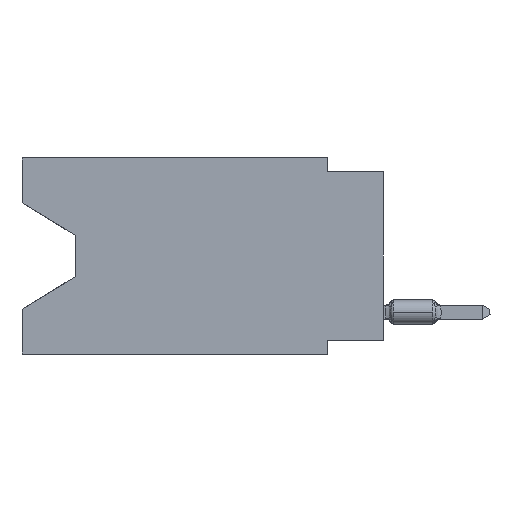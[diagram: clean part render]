
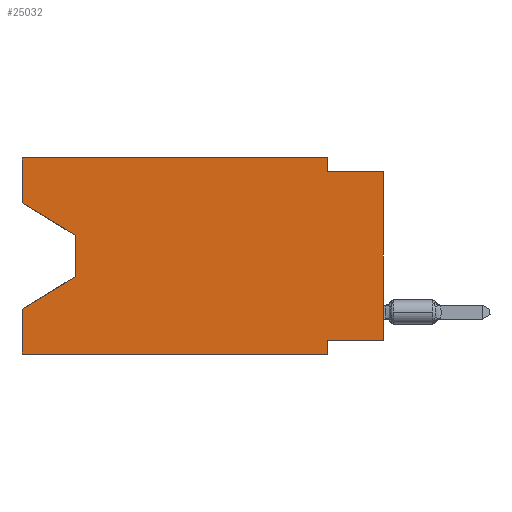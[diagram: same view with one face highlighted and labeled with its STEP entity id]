
A CAD part, left-side view. The second image highlights one B-rep face of the part: STEP entity #25032.
In plain terms, the highlighted planar face has unit normal (-1, 0, 0).
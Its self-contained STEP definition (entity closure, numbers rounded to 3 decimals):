
#564 = ORIENTED_EDGE ( 'NONE', *, *, #35363, .F. ) ;
#917 = CARTESIAN_POINT ( 'NONE',  ( 0., 0., -0.635 ) ) ;
#2523 = VERTEX_POINT ( 'NONE', #16397 ) ;
#2773 = VERTEX_POINT ( 'NONE', #14297 ) ;
#3622 = DIRECTION ( 'NONE',  ( 0., 0., -1. ) ) ;
#4265 = DIRECTION ( 'NONE',  ( 0., 0., -1. ) ) ;
#4941 = EDGE_CURVE ( 'NONE', #18006, #2773, #11663, .T. ) ;
#5604 = EDGE_CURVE ( 'NONE', #17813, #47537, #65028, .T. ) ;
#5994 = AXIS2_PLACEMENT_3D ( 'NONE', #54937, #60303, #4265 ) ;
#6298 = DIRECTION ( 'NONE',  ( 0., 0., -1. ) ) ;
#6953 = DIRECTION ( 'NONE',  ( 0., 0., 1. ) ) ;
#7023 = EDGE_CURVE ( 'NONE', #32067, #2523, #47996, .T. ) ;
#8337 = EDGE_CURVE ( 'NONE', #59845, #60852, #10118, .T. ) ;
#9528 = VECTOR ( 'NONE', #43289, 1000. ) ;
#9959 = VECTOR ( 'NONE', #50485, 1000. ) ;
#10118 = LINE ( 'NONE', #11137, #41432 ) ;
#10743 = EDGE_CURVE ( 'NONE', #2523, #35669, #17047, .T. ) ;
#11085 = DIRECTION ( 'NONE',  ( 0., -1., 0. ) ) ;
#11137 = CARTESIAN_POINT ( 'NONE',  ( 0., 16.383, 0. ) ) ;
#11663 = LINE ( 'NONE', #31842, #63995 ) ;
#11842 = ORIENTED_EDGE ( 'NONE', *, *, #14640, .T. ) ;
#12755 = CARTESIAN_POINT ( 'NONE',  ( 0., 13.97, -3.505 ) ) ;
#14036 = CARTESIAN_POINT ( 'NONE',  ( 0., 2.54, -8.89 ) ) ;
#14253 = CARTESIAN_POINT ( 'NONE',  ( 0., 16.383, -2.038 ) ) ;
#14297 = CARTESIAN_POINT ( 'NONE',  ( 0., 16.383, -6.852 ) ) ;
#14640 = EDGE_CURVE ( 'NONE', #47634, #35669, #22160, .T. ) ;
#15418 = EDGE_CURVE ( 'NONE', #40428, #2773, #18667, .T. ) ;
#16397 = CARTESIAN_POINT ( 'NONE',  ( 0., 2.54, -0.635 ) ) ;
#16847 = CARTESIAN_POINT ( 'NONE',  ( 0., 13.97, -5.385 ) ) ;
#17047 = LINE ( 'NONE', #917, #25531 ) ;
#17813 = VERTEX_POINT ( 'NONE', #23313 ) ;
#18006 = VERTEX_POINT ( 'NONE', #44403 ) ;
#18667 = LINE ( 'NONE', #55518, #9959 ) ;
#20859 = LINE ( 'NONE', #32596, #36740 ) ;
#22106 = LINE ( 'NONE', #32823, #47673 ) ;
#22160 = LINE ( 'NONE', #37249, #54648 ) ;
#22765 = DIRECTION ( 'NONE',  ( 0., -1., 0. ) ) ;
#23313 = CARTESIAN_POINT ( 'NONE',  ( 0., 2.54, -8.255 ) ) ;
#25032 = ADVANCED_FACE ( 'NONE', ( #45218 ), #55597, .F. ) ;
#25205 = ORIENTED_EDGE ( 'NONE', *, *, #28951, .F. ) ;
#25531 = VECTOR ( 'NONE', #22765, 1000. ) ;
#28951 = EDGE_CURVE ( 'NONE', #47634, #17813, #66301, .T. ) ;
#30199 = CARTESIAN_POINT ( 'NONE',  ( 0., 0., -0.635 ) ) ;
#30381 = LINE ( 'NONE', #14253, #64948 ) ;
#30484 = ORIENTED_EDGE ( 'NONE', *, *, #15418, .T. ) ;
#31383 = CARTESIAN_POINT ( 'NONE',  ( 0., 0., -8.255 ) ) ;
#31407 = ORIENTED_EDGE ( 'NONE', *, *, #8337, .F. ) ;
#31522 = ORIENTED_EDGE ( 'NONE', *, *, #55062, .T. ) ;
#31842 = CARTESIAN_POINT ( 'NONE',  ( 0., 16.383, 0. ) ) ;
#32067 = VERTEX_POINT ( 'NONE', #64496 ) ;
#32596 = CARTESIAN_POINT ( 'NONE',  ( 0., 16.383, 0. ) ) ;
#32823 = CARTESIAN_POINT ( 'NONE',  ( 0., 13.97, -3.505 ) ) ;
#33250 = VECTOR ( 'NONE', #60283, 1000. ) ;
#34015 = ORIENTED_EDGE ( 'NONE', *, *, #7023, .F. ) ;
#35363 = EDGE_CURVE ( 'NONE', #60852, #32067, #20859, .T. ) ;
#35669 = VERTEX_POINT ( 'NONE', #30199 ) ;
#36375 = ORIENTED_EDGE ( 'NONE', *, *, #10743, .F. ) ;
#36387 = ORIENTED_EDGE ( 'NONE', *, *, #5604, .F. ) ;
#36740 = VECTOR ( 'NONE', #11085, 1000. ) ;
#37249 = CARTESIAN_POINT ( 'NONE',  ( 0., 0., 0. ) ) ;
#37597 = LINE ( 'NONE', #58042, #9528 ) ;
#37730 = CARTESIAN_POINT ( 'NONE',  ( 0., 16.383, 0. ) ) ;
#38500 = VECTOR ( 'NONE', #3622, 1000. ) ;
#40428 = VERTEX_POINT ( 'NONE', #16847 ) ;
#40830 = CARTESIAN_POINT ( 'NONE',  ( 0., 0., -8.255 ) ) ;
#41432 = VECTOR ( 'NONE', #47410, 1000. ) ;
#42965 = CARTESIAN_POINT ( 'NONE',  ( 0., 2.54, 0. ) ) ;
#43289 = DIRECTION ( 'NONE',  ( 0., -1., 0. ) ) ;
#43401 = ORIENTED_EDGE ( 'NONE', *, *, #4941, .F. ) ;
#43873 = ORIENTED_EDGE ( 'NONE', *, *, #47432, .T. ) ;
#44403 = CARTESIAN_POINT ( 'NONE',  ( 0., 16.383, -8.89 ) ) ;
#45218 = FACE_OUTER_BOUND ( 'NONE', #49622, .T. ) ;
#46239 = EDGE_CURVE ( 'NONE', #46927, #40428, #22106, .T. ) ;
#46927 = VERTEX_POINT ( 'NONE', #12755 ) ;
#47144 = CARTESIAN_POINT ( 'NONE',  ( 0., 2.54, -8.89 ) ) ;
#47263 = VECTOR ( 'NONE', #63410, 1000. ) ;
#47312 = DIRECTION ( 'NONE',  ( 0., 0., 1. ) ) ;
#47410 = DIRECTION ( 'NONE',  ( 0., 0., 1. ) ) ;
#47432 = EDGE_CURVE ( 'NONE', #59845, #46927, #30381, .T. ) ;
#47537 = VERTEX_POINT ( 'NONE', #47144 ) ;
#47634 = VERTEX_POINT ( 'NONE', #31383 ) ;
#47673 = VECTOR ( 'NONE', #6298, 1000. ) ;
#47996 = LINE ( 'NONE', #42965, #47263 ) ;
#49622 = EDGE_LOOP ( 'NONE', ( #43873, #57104, #30484, #43401, #31522, #36387, #25205, #11842, #36375, #34015, #564, #31407 ) ) ;
#49697 = CARTESIAN_POINT ( 'NONE',  ( 0., 16.383, -2.038 ) ) ;
#50485 = DIRECTION ( 'NONE',  ( 0., 0.855, -0.519 ) ) ;
#50804 = DIRECTION ( 'NONE',  ( 0., -0.855, -0.519 ) ) ;
#54648 = VECTOR ( 'NONE', #47312, 1000. ) ;
#54937 = CARTESIAN_POINT ( 'NONE',  ( 0., 16.383, 0. ) ) ;
#55062 = EDGE_CURVE ( 'NONE', #18006, #47537, #37597, .T. ) ;
#55518 = CARTESIAN_POINT ( 'NONE',  ( 0., 13.97, -5.385 ) ) ;
#55597 = PLANE ( 'NONE',  #5994 ) ;
#57104 = ORIENTED_EDGE ( 'NONE', *, *, #46239, .T. ) ;
#58042 = CARTESIAN_POINT ( 'NONE',  ( 0., 16.383, -8.89 ) ) ;
#59845 = VERTEX_POINT ( 'NONE', #49697 ) ;
#60283 = DIRECTION ( 'NONE',  ( 0., 1., 0. ) ) ;
#60303 = DIRECTION ( 'NONE',  ( 1., 0., 0. ) ) ;
#60852 = VERTEX_POINT ( 'NONE', #37730 ) ;
#63410 = DIRECTION ( 'NONE',  ( 0., 0., -1. ) ) ;
#63995 = VECTOR ( 'NONE', #6953, 1000. ) ;
#64496 = CARTESIAN_POINT ( 'NONE',  ( 0., 2.54, 0. ) ) ;
#64948 = VECTOR ( 'NONE', #50804, 1000. ) ;
#65028 = LINE ( 'NONE', #14036, #38500 ) ;
#66301 = LINE ( 'NONE', #40830, #33250 ) ;
